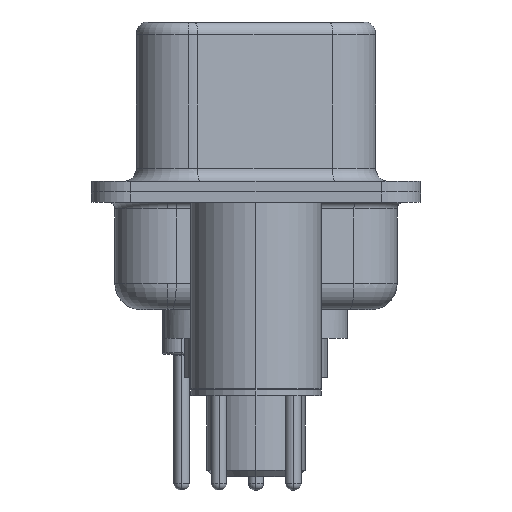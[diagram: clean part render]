
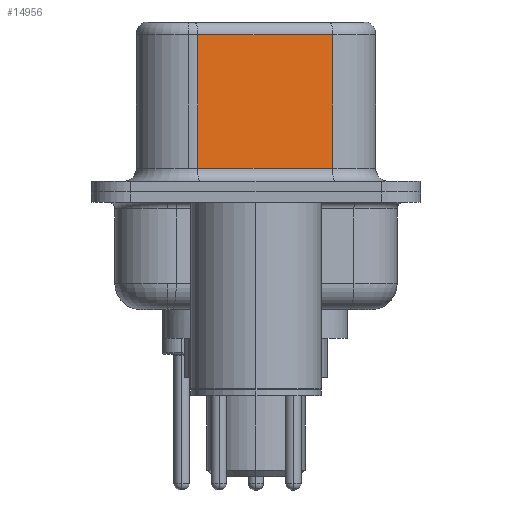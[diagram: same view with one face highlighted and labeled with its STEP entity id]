
A CAD part, left-side view. The second image highlights one B-rep face of the part: STEP entity #14956.
In plain terms, the highlighted planar face has unit normal (-0.985, -0.174, 0).
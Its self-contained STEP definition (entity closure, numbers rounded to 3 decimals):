
#132 = CARTESIAN_POINT ( 'NONE',  ( 4.585, -2.927, 6.02 ) ) ;
#944 = CARTESIAN_POINT ( 'NONE',  ( 4.585, -2.927, 6.02 ) ) ;
#1848 = DIRECTION ( 'NONE',  ( 0.174, -0.985, 0. ) ) ;
#3218 = EDGE_CURVE ( 'NONE', #17690, #7386, #13986, .T. ) ;
#4299 = AXIS2_PLACEMENT_3D ( 'NONE', #20961, #18869, #16881 ) ;
#5018 = CARTESIAN_POINT ( 'NONE',  ( 4.585, -2.927, 0.9 ) ) ;
#6056 = VECTOR ( 'NONE', #1848, 1000. ) ;
#7125 = EDGE_CURVE ( 'NONE', #12260, #7386, #17696, .T. ) ;
#7386 = VERTEX_POINT ( 'NONE', #5018 ) ;
#7923 = DIRECTION ( 'NONE',  ( 0., 0., -1. ) ) ;
#8658 = DIRECTION ( 'NONE',  ( 0., 0., -1. ) ) ;
#9070 = CARTESIAN_POINT ( 'NONE',  ( 3.675, 2.233, 0.9 ) ) ;
#9888 = LINE ( 'NONE', #944, #13464 ) ;
#10256 = EDGE_CURVE ( 'NONE', #17690, #13972, #9888, .T. ) ;
#11990 = ORIENTED_EDGE ( 'NONE', *, *, #3218, .F. ) ;
#12260 = VERTEX_POINT ( 'NONE', #9070 ) ;
#12373 = LINE ( 'NONE', #18281, #21929 ) ;
#12704 = ORIENTED_EDGE ( 'NONE', *, *, #16037, .T. ) ;
#13021 = FACE_OUTER_BOUND ( 'NONE', #17929, .T. ) ;
#13464 = VECTOR ( 'NONE', #20106, 1000. ) ;
#13972 = VERTEX_POINT ( 'NONE', #15011 ) ;
#13986 = LINE ( 'NONE', #21227, #20277 ) ;
#14163 = ORIENTED_EDGE ( 'NONE', *, *, #10256, .T. ) ;
#14956 = ADVANCED_FACE ( 'NONE', ( #13021 ), #15113, .F. ) ;
#15011 = CARTESIAN_POINT ( 'NONE',  ( 3.675, 2.233, 6.02 ) ) ;
#15113 = PLANE ( 'NONE',  #4299 ) ;
#16037 = EDGE_CURVE ( 'NONE', #13972, #12260, #12373, .T. ) ;
#16881 = DIRECTION ( 'NONE',  ( -0.174, 0.985, 0. ) ) ;
#17690 = VERTEX_POINT ( 'NONE', #132 ) ;
#17696 = LINE ( 'NONE', #23168, #6056 ) ;
#17929 = EDGE_LOOP ( 'NONE', ( #11990, #14163, #12704, #18871 ) ) ;
#18281 = CARTESIAN_POINT ( 'NONE',  ( 3.675, 2.233, 6.52 ) ) ;
#18869 = DIRECTION ( 'NONE',  ( 0.985, 0.174, 0. ) ) ;
#18871 = ORIENTED_EDGE ( 'NONE', *, *, #7125, .T. ) ;
#20106 = DIRECTION ( 'NONE',  ( -0.174, 0.985, 0. ) ) ;
#20277 = VECTOR ( 'NONE', #7923, 1000. ) ;
#20961 = CARTESIAN_POINT ( 'NONE',  ( 4.585, -2.927, 6.52 ) ) ;
#21227 = CARTESIAN_POINT ( 'NONE',  ( 4.585, -2.927, 6.52 ) ) ;
#21929 = VECTOR ( 'NONE', #8658, 1000. ) ;
#23168 = CARTESIAN_POINT ( 'NONE',  ( 4.585, -2.927, 0.9 ) ) ;
